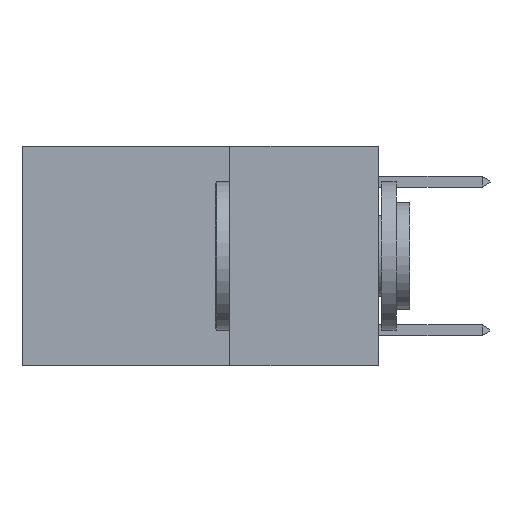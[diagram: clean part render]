
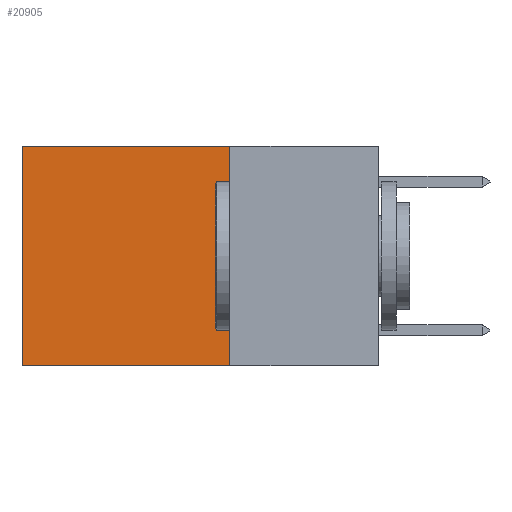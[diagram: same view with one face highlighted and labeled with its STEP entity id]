
A CAD part, left-side view. The second image highlights one B-rep face of the part: STEP entity #20905.
In plain terms, the highlighted planar face has unit normal (-1, 0, 0).
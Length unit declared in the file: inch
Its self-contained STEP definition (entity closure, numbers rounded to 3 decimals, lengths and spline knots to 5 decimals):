
#306 = VECTOR ( 'NONE', #9163, 39.37008 ) ;
#1010 = CARTESIAN_POINT ( 'NONE',  ( 0.2625, 0.25, -0.37 ) ) ;
#2848 = VECTOR ( 'NONE', #23742, 39.37008 ) ;
#3750 = PLANE ( 'NONE',  #11786 ) ;
#4179 = VERTEX_POINT ( 'NONE', #28732 ) ;
#5664 = CARTESIAN_POINT ( 'NONE',  ( 0.2625, 0.25, 0. ) ) ;
#5708 = LINE ( 'NONE', #22756, #306 ) ;
#7153 = DIRECTION ( 'NONE',  ( 0., 0., -1. ) ) ;
#8158 = LINE ( 'NONE', #1010, #2848 ) ;
#8404 = CARTESIAN_POINT ( 'NONE',  ( 0.2625, 0.25, 0. ) ) ;
#8605 = VECTOR ( 'NONE', #7153, 39.37008 ) ;
#8708 = VERTEX_POINT ( 'NONE', #11455 ) ;
#9163 = DIRECTION ( 'NONE',  ( 0., 0., -1. ) ) ;
#9641 = VECTOR ( 'NONE', #14593, 39.37008 ) ;
#10643 = DIRECTION ( 'NONE',  ( 0., 0., -1. ) ) ;
#11455 = CARTESIAN_POINT ( 'NONE',  ( 0.2625, 0.25, -0.37 ) ) ;
#11786 = AXIS2_PLACEMENT_3D ( 'NONE', #8404, #24251, #10643 ) ;
#12216 = CARTESIAN_POINT ( 'NONE',  ( 0.2625, 0.25, 0. ) ) ;
#14593 = DIRECTION ( 'NONE',  ( 0., 1., 0. ) ) ;
#17120 = FACE_OUTER_BOUND ( 'NONE', #27046, .T. ) ;
#20314 = CARTESIAN_POINT ( 'NONE',  ( 0.2625, 0.6, -0.37 ) ) ;
#20905 = ADVANCED_FACE ( 'NONE', ( #17120 ), #3750, .F. ) ;
#20995 = ORIENTED_EDGE ( 'NONE', *, *, #23207, .F. ) ;
#21729 = LINE ( 'NONE', #5664, #9641 ) ;
#22073 = VERTEX_POINT ( 'NONE', #12216 ) ;
#22122 = EDGE_CURVE ( 'NONE', #22073, #4179, #21729, .T. ) ;
#22242 = ORIENTED_EDGE ( 'NONE', *, *, #28395, .T. ) ;
#22485 = VERTEX_POINT ( 'NONE', #20314 ) ;
#22756 = CARTESIAN_POINT ( 'NONE',  ( 0.2625, 0.25, 0. ) ) ;
#23068 = ORIENTED_EDGE ( 'NONE', *, *, #22122, .T. ) ;
#23207 = EDGE_CURVE ( 'NONE', #22073, #8708, #5708, .T. ) ;
#23742 = DIRECTION ( 'NONE',  ( 0., 1., 0. ) ) ;
#23793 = EDGE_CURVE ( 'NONE', #8708, #22485, #8158, .T. ) ;
#24251 = DIRECTION ( 'NONE',  ( 1., 0., 0. ) ) ;
#25275 = CARTESIAN_POINT ( 'NONE',  ( 0.2625, 0.6, 0. ) ) ;
#25774 = ORIENTED_EDGE ( 'NONE', *, *, #23793, .F. ) ;
#27046 = EDGE_LOOP ( 'NONE', ( #22242, #25774, #20995, #23068 ) ) ;
#27398 = LINE ( 'NONE', #25275, #8605 ) ;
#28395 = EDGE_CURVE ( 'NONE', #4179, #22485, #27398, .T. ) ;
#28732 = CARTESIAN_POINT ( 'NONE',  ( 0.2625, 0.6, 0. ) ) ;
